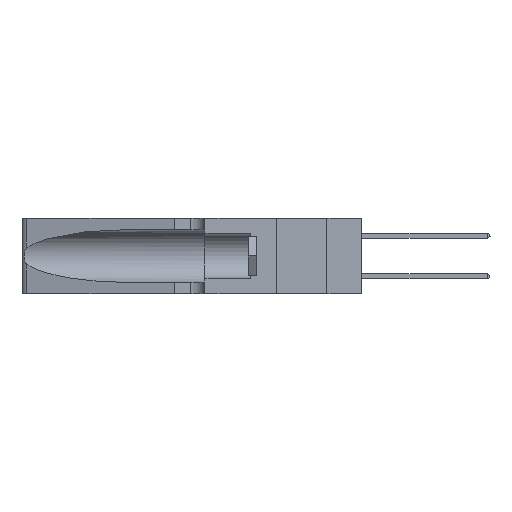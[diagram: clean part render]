
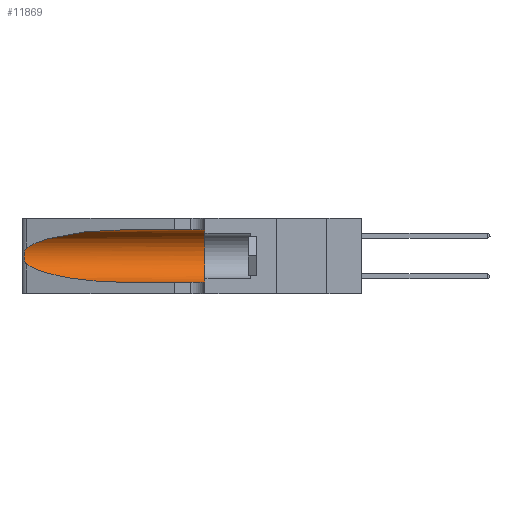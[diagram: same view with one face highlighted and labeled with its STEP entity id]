
A CAD part, left-side view. The second image highlights one B-rep face of the part: STEP entity #11869.
In plain terms, the highlighted cylindrical face has radius 3.308 mm (diameter 6.617 mm), a partial arc.
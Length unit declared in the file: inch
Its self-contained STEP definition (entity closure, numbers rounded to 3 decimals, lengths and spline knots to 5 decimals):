
#205 = ORIENTED_EDGE ( 'NONE', *, *, #43688, .T. ) ;
#477 = CARTESIAN_POINT ( 'NONE',  ( 0.25787, 1.23484, 0.2124 ) ) ;
#1860 = VERTEX_POINT ( 'NONE', #13577 ) ;
#2902 = CARTESIAN_POINT ( 'NONE',  ( 0.1305, 0.35, 0.31525 ) ) ;
#4026 = CARTESIAN_POINT ( 'NONE',  ( 0.26018, 1.23835, 0.19895 ) ) ;
#5051 = VERTEX_POINT ( 'NONE', #38490 ) ;
#6717 = CYLINDRICAL_SURFACE ( 'NONE', #16605, 0.13025 ) ;
#7145 = CARTESIAN_POINT ( 'NONE',  ( 0.25487, 1.22718, 0.22369 ) ) ;
#7581 = CARTESIAN_POINT ( 'NONE',  ( 0.26075, 1.23896, 0.178 ) ) ;
#7865 = FACE_OUTER_BOUND ( 'NONE', #37373, .T. ) ;
#9813 = CARTESIAN_POINT ( 'NONE',  ( 0.2373, 1.15595, 0.08982 ) ) ;
#10188 = EDGE_CURVE ( 'NONE', #1860, #30713, #19007, .T. ) ;
#10984 = CARTESIAN_POINT ( 'NONE',  ( 0.25487, 1.22718, 0.22369 ) ) ;
#11145 = CARTESIAN_POINT ( 'NONE',  ( 0.25856, 1.23593, 0.16098 ) ) ;
#11869 = ADVANCED_FACE ( 'NONE', ( #7865 ), #6717, .F. ) ;
#12455 = CIRCLE ( 'NONE', #13197, 0.13025 ) ;
#12570 = DIRECTION ( 'NONE',  ( 0., -1., 0. ) ) ;
#12574 = CARTESIAN_POINT ( 'NONE',  ( 0.1305, 1.61858, 0.185 ) ) ;
#12950 = ORIENTED_EDGE ( 'NONE', *, *, #43058, .F. ) ;
#13175 = CARTESIAN_POINT ( 'NONE',  ( 0.25487, 1.22718, 0.22369 ) ) ;
#13197 = AXIS2_PLACEMENT_3D ( 'NONE', #37324, #16638, #40787 ) ;
#13208 = CARTESIAN_POINT ( 'NONE',  ( 0.25487, 1.22718, 0.14631 ) ) ;
#13577 = CARTESIAN_POINT ( 'NONE',  ( 0.1305, 0.72297, 0.31525 ) ) ;
#14585 = ORIENTED_EDGE ( 'NONE', *, *, #33662, .T. ) ;
#14708 = CARTESIAN_POINT ( 'NONE',  ( 0.25639, 1.23186, 0.15144 ) ) ;
#16605 = AXIS2_PLACEMENT_3D ( 'NONE', #12574, #19461, #22952 ) ;
#16638 = DIRECTION ( 'NONE',  ( 0., 1., 0. ) ) ;
#16894 = CARTESIAN_POINT ( 'NONE',  ( 0.1305, 0.72297, 0.05475 ) ) ;
#17629 = CARTESIAN_POINT ( 'NONE',  ( 0.1305, 0.35, 0.05475 ) ) ;
#18119 = B_SPLINE_CURVE_WITH_KNOTS ( 'NONE', 3,
 ( #10984, #31791, #21554, #477, #25025, #4026, #28485, #7581, #31947, #11145, #35423, #14708, #38909, #18222 ),
 .UNSPECIFIED., .F., .F.,
 ( 4, 2, 2, 2, 2, 2, 4 ),
 ( 0., 0.00027, 0.00053, 0.00107, 0.0016, 0.00187, 0.00214 ),
 .UNSPECIFIED. ) ;
#18222 = CARTESIAN_POINT ( 'NONE',  ( 0.25487, 1.22718, 0.14631 ) ) ;
#19000 = VERTEX_POINT ( 'NONE', #17629 ) ;
#19007 = LINE ( 'NONE', #28039, #36303 ) ;
#19461 = DIRECTION ( 'NONE',  ( 0., -1., 0. ) ) ;
#19700 = CARTESIAN_POINT ( 'NONE',  ( 0.1305, 0.72297, 0.05475 ) ) ;
#21059 = EDGE_CURVE ( 'NONE', #27379, #5051, #18119, .T. ) ;
#21554 = CARTESIAN_POINT ( 'NONE',  ( 0.25639, 1.23184, 0.21858 ) ) ;
#22243 = ORIENTED_EDGE ( 'NONE', *, *, #10188, .F. ) ;
#22952 = DIRECTION ( 'NONE',  ( 0., 0., -1. ) ) ;
#23537 = CARTESIAN_POINT ( 'NONE',  ( 0.1305, 0.72297, 0.31525 ) ) ;
#25025 = CARTESIAN_POINT ( 'NONE',  ( 0.25854, 1.2359, 0.20912 ) ) ;
#26661 = LINE ( 'NONE', #43576, #35839 ) ;
#27379 = VERTEX_POINT ( 'NONE', #7145 ) ;
#28039 = CARTESIAN_POINT ( 'NONE',  ( 0.1305, 1.61858, 0.31525 ) ) ;
#28485 = CARTESIAN_POINT ( 'NONE',  ( 0.26075, 1.23896, 0.19203 ) ) ;
#30713 = VERTEX_POINT ( 'NONE', #2902 ) ;
#30839 =( BOUNDED_CURVE ( )  B_SPLINE_CURVE ( 3, ( #23537, #44147, #33929, #13175 ),
 .UNSPECIFIED., .F., .F. ) 
 B_SPLINE_CURVE_WITH_KNOTS ( ( 4, 4 ),
 ( 1.5708, 2.84003 ),
 .UNSPECIFIED. ) 
 CURVE ( )  GEOMETRIC_REPRESENTATION_ITEM ( )  RATIONAL_B_SPLINE_CURVE ( ( 1., 0.87, 0.87, 1. ) ) 
 REPRESENTATION_ITEM ( '' )  );
#31493 = DIRECTION ( 'NONE',  ( 0., -1., 0. ) ) ;
#31791 = CARTESIAN_POINT ( 'NONE',  ( 0.25555, 1.22994, 0.2215 ) ) ;
#31947 = CARTESIAN_POINT ( 'NONE',  ( 0.26017, 1.23833, 0.17102 ) ) ;
#33662 = EDGE_CURVE ( 'NONE', #1860, #27379, #30839, .T. ) ;
#33929 = CARTESIAN_POINT ( 'NONE',  ( 0.2373, 1.15595, 0.28018 ) ) ;
#35423 = CARTESIAN_POINT ( 'NONE',  ( 0.25789, 1.23486, 0.15765 ) ) ;
#35566 =( BOUNDED_CURVE ( )  B_SPLINE_CURVE ( 3, ( #13208, #9813, #37560, #16894 ),
 .UNSPECIFIED., .F., .F. ) 
 B_SPLINE_CURVE_WITH_KNOTS ( ( 4, 4 ),
 ( 3.44316, 4.71239 ),
 .UNSPECIFIED. ) 
 CURVE ( )  GEOMETRIC_REPRESENTATION_ITEM ( )  RATIONAL_B_SPLINE_CURVE ( ( 1., 0.87, 0.87, 1. ) ) 
 REPRESENTATION_ITEM ( '' )  );
#35839 = VECTOR ( 'NONE', #12570, 39.37008 ) ;
#36262 = ORIENTED_EDGE ( 'NONE', *, *, #21059, .T. ) ;
#36303 = VECTOR ( 'NONE', #31493, 39.37008 ) ;
#37324 = CARTESIAN_POINT ( 'NONE',  ( 0.1305, 0.35, 0.185 ) ) ;
#37373 = EDGE_LOOP ( 'NONE', ( #14585, #36262, #205, #39492, #12950, #22243 ) ) ;
#37560 = CARTESIAN_POINT ( 'NONE',  ( 0.18966, 0.96281, 0.05475 ) ) ;
#38490 = CARTESIAN_POINT ( 'NONE',  ( 0.25487, 1.22718, 0.14631 ) ) ;
#38909 = CARTESIAN_POINT ( 'NONE',  ( 0.25555, 1.22993, 0.14849 ) ) ;
#39492 = ORIENTED_EDGE ( 'NONE', *, *, #42732, .T. ) ;
#39851 = VERTEX_POINT ( 'NONE', #19700 ) ;
#40787 = DIRECTION ( 'NONE',  ( 0., 0., 1. ) ) ;
#42732 = EDGE_CURVE ( 'NONE', #39851, #19000, #26661, .T. ) ;
#43058 = EDGE_CURVE ( 'NONE', #30713, #19000, #12455, .T. ) ;
#43576 = CARTESIAN_POINT ( 'NONE',  ( 0.1305, 1.61858, 0.05475 ) ) ;
#43688 = EDGE_CURVE ( 'NONE', #5051, #39851, #35566, .T. ) ;
#44147 = CARTESIAN_POINT ( 'NONE',  ( 0.18966, 0.96281, 0.31525 ) ) ;
